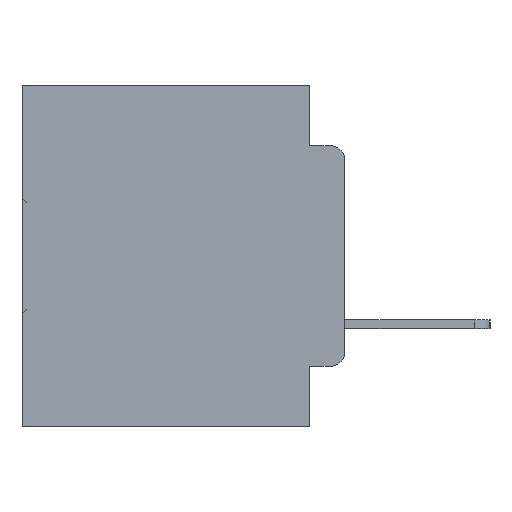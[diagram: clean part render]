
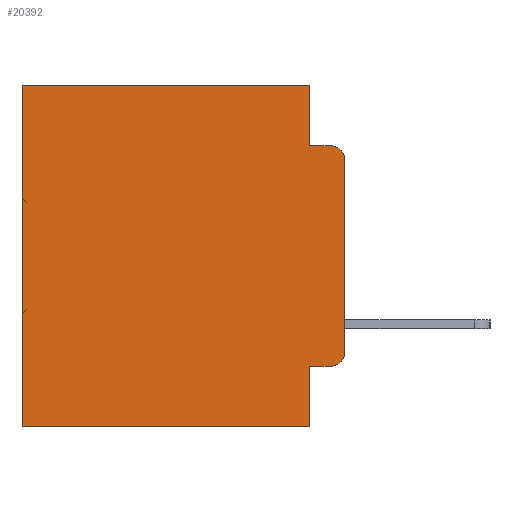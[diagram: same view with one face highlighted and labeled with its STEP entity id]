
A CAD part, left-side view. The second image highlights one B-rep face of the part: STEP entity #20392.
In plain terms, the highlighted planar face has unit normal (-1, 0, 0).
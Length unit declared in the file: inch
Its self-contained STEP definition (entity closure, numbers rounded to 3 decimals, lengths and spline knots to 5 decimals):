
#86 = DIRECTION ( 'NONE',  ( 0., -1., 0. ) ) ;
#613 = VERTEX_POINT ( 'NONE', #7972 ) ;
#655 = CARTESIAN_POINT ( 'NONE',  ( 0.298, 0.051, 0. ) ) ;
#711 = DIRECTION ( 'NONE',  ( 0., 1., 0. ) ) ;
#778 = VECTOR ( 'NONE', #26476, 39.37008 ) ;
#1637 = VERTEX_POINT ( 'NONE', #27087 ) ;
#1897 = CIRCLE ( 'NONE', #25636, 0.02 ) ;
#1906 = CARTESIAN_POINT ( 'NONE',  ( 0.298, 0.02, -0.1085 ) ) ;
#2430 = CARTESIAN_POINT ( 'NONE',  ( 0.298, 0.051, -0.0885 ) ) ;
#2504 = LINE ( 'NONE', #7860, #16029 ) ;
#2678 = VECTOR ( 'NONE', #33450, 39.37008 ) ;
#3365 = DIRECTION ( 'NONE',  ( 0., 0., -1. ) ) ;
#3537 = LINE ( 'NONE', #4108, #2678 ) ;
#3845 = VERTEX_POINT ( 'NONE', #28369 ) ;
#3922 = ORIENTED_EDGE ( 'NONE', *, *, #25397, .T. ) ;
#4108 = CARTESIAN_POINT ( 'NONE',  ( 0.298, 0.473, 0. ) ) ;
#4537 = CARTESIAN_POINT ( 'NONE',  ( 0.298, 0.02, -0.4115 ) ) ;
#4602 = DIRECTION ( 'NONE',  ( 0., 0., -1. ) ) ;
#5929 = ORIENTED_EDGE ( 'NONE', *, *, #30091, .T. ) ;
#6422 = CARTESIAN_POINT ( 'NONE',  ( 0.298, 0.473, -0.5 ) ) ;
#6531 = ORIENTED_EDGE ( 'NONE', *, *, #10881, .F. ) ;
#7198 = LINE ( 'NONE', #655, #21513 ) ;
#7860 = CARTESIAN_POINT ( 'NONE',  ( 0.298, 0.051, -0.0885 ) ) ;
#7970 = DIRECTION ( 'NONE',  ( 0., -1., 0. ) ) ;
#7972 = CARTESIAN_POINT ( 'NONE',  ( 0.298, 0.02, -0.0885 ) ) ;
#8628 = VECTOR ( 'NONE', #86, 39.37008 ) ;
#8663 = ORIENTED_EDGE ( 'NONE', *, *, #32930, .F. ) ;
#9893 = AXIS2_PLACEMENT_3D ( 'NONE', #14852, #33451, #17573 ) ;
#10376 = CARTESIAN_POINT ( 'NONE',  ( 0.298, 0., 0. ) ) ;
#10881 = EDGE_CURVE ( 'NONE', #1637, #14775, #29240, .T. ) ;
#11118 = ORIENTED_EDGE ( 'NONE', *, *, #17186, .F. ) ;
#11162 = ORIENTED_EDGE ( 'NONE', *, *, #12174, .T. ) ;
#11451 = CARTESIAN_POINT ( 'NONE',  ( 0.298, 0., 0. ) ) ;
#11669 = VECTOR ( 'NONE', #32351, 39.37008 ) ;
#12174 = EDGE_CURVE ( 'NONE', #23349, #15529, #29955, .T. ) ;
#12830 = FACE_OUTER_BOUND ( 'NONE', #18153, .T. ) ;
#12940 = DIRECTION ( 'NONE',  ( -1., 0., 0. ) ) ;
#13095 = CARTESIAN_POINT ( 'NONE',  ( 0.298, 0.051, 0. ) ) ;
#14184 = AXIS2_PLACEMENT_3D ( 'NONE', #28961, #12940, #31580 ) ;
#14388 = VERTEX_POINT ( 'NONE', #23439 ) ;
#14775 = VERTEX_POINT ( 'NONE', #22509 ) ;
#14852 = CARTESIAN_POINT ( 'NONE',  ( 0.298, 0., 0. ) ) ;
#14910 = EDGE_CURVE ( 'NONE', #14388, #15997, #3537, .T. ) ;
#15031 = VECTOR ( 'NONE', #34394, 39.37008 ) ;
#15166 = LINE ( 'NONE', #11451, #28564 ) ;
#15529 = VERTEX_POINT ( 'NONE', #4537 ) ;
#15997 = VERTEX_POINT ( 'NONE', #6422 ) ;
#16029 = VECTOR ( 'NONE', #7970, 39.37008 ) ;
#16134 = CIRCLE ( 'NONE', #14184, 0.02 ) ;
#17186 = EDGE_CURVE ( 'NONE', #23349, #3845, #7198, .T. ) ;
#17573 = DIRECTION ( 'NONE',  ( 0., 0., -1. ) ) ;
#18153 = EDGE_LOOP ( 'NONE', ( #6531, #25370, #29115, #20396, #3922, #23410, #8663, #11118, #11162, #5929 ) ) ;
#19884 = EDGE_CURVE ( 'NONE', #1637, #613, #1897, .T. ) ;
#20392 = ADVANCED_FACE ( 'NONE', ( #12830 ), #30807, .F. ) ;
#20396 = ORIENTED_EDGE ( 'NONE', *, *, #23939, .F. ) ;
#20789 = DIRECTION ( 'NONE',  ( -1., 0., 0. ) ) ;
#21513 = VECTOR ( 'NONE', #3365, 39.37008 ) ;
#22509 = CARTESIAN_POINT ( 'NONE',  ( 0.298, 0., -0.3915 ) ) ;
#23349 = VERTEX_POINT ( 'NONE', #33872 ) ;
#23410 = ORIENTED_EDGE ( 'NONE', *, *, #14910, .T. ) ;
#23439 = CARTESIAN_POINT ( 'NONE',  ( 0.298, 0.473, 0. ) ) ;
#23473 = EDGE_CURVE ( 'NONE', #32146, #613, #2504, .T. ) ;
#23939 = EDGE_CURVE ( 'NONE', #30735, #32146, #28530, .T. ) ;
#25370 = ORIENTED_EDGE ( 'NONE', *, *, #19884, .T. ) ;
#25397 = EDGE_CURVE ( 'NONE', #30735, #14388, #15166, .T. ) ;
#25636 = AXIS2_PLACEMENT_3D ( 'NONE', #1906, #20789, #4602 ) ;
#26476 = DIRECTION ( 'NONE',  ( 0., 0., -1. ) ) ;
#27087 = CARTESIAN_POINT ( 'NONE',  ( 0.298, 0., -0.1085 ) ) ;
#27215 = CARTESIAN_POINT ( 'NONE',  ( 0.298, 0., -0.5 ) ) ;
#28369 = CARTESIAN_POINT ( 'NONE',  ( 0.298, 0.051, -0.5 ) ) ;
#28474 = CARTESIAN_POINT ( 'NONE',  ( 0.298, 0.051, 0. ) ) ;
#28530 = LINE ( 'NONE', #13095, #778 ) ;
#28564 = VECTOR ( 'NONE', #711, 39.37008 ) ;
#28961 = CARTESIAN_POINT ( 'NONE',  ( 0.298, 0.02, -0.3915 ) ) ;
#29115 = ORIENTED_EDGE ( 'NONE', *, *, #23473, .F. ) ;
#29240 = LINE ( 'NONE', #10376, #15031 ) ;
#29955 = LINE ( 'NONE', #32204, #8628 ) ;
#30091 = EDGE_CURVE ( 'NONE', #15529, #14775, #16134, .T. ) ;
#30735 = VERTEX_POINT ( 'NONE', #28474 ) ;
#30807 = PLANE ( 'NONE',  #9893 ) ;
#31580 = DIRECTION ( 'NONE',  ( 0., 0., -1. ) ) ;
#32146 = VERTEX_POINT ( 'NONE', #2430 ) ;
#32204 = CARTESIAN_POINT ( 'NONE',  ( 0.298, 0.051, -0.4115 ) ) ;
#32351 = DIRECTION ( 'NONE',  ( 0., 1., 0. ) ) ;
#32930 = EDGE_CURVE ( 'NONE', #3845, #15997, #32956, .T. ) ;
#32956 = LINE ( 'NONE', #27215, #11669 ) ;
#33450 = DIRECTION ( 'NONE',  ( 0., 0., -1. ) ) ;
#33451 = DIRECTION ( 'NONE',  ( 1., 0., 0. ) ) ;
#33872 = CARTESIAN_POINT ( 'NONE',  ( 0.298, 0.051, -0.4115 ) ) ;
#34394 = DIRECTION ( 'NONE',  ( 0., 0., -1. ) ) ;
